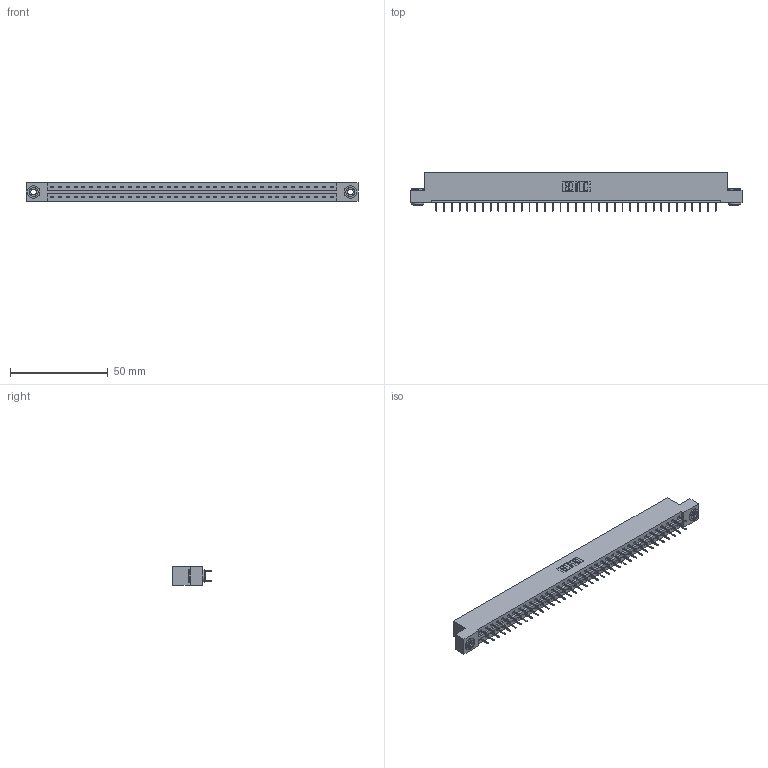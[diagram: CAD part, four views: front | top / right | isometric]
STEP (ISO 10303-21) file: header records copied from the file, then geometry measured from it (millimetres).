
FILE_DESCRIPTION (( 'STEP AP203' ), '1' );
FILE_NAME ('387-074-524-203.STEP', '2018-09-22T19:36:12', ( '' ), ( '' ), 'SwSTEP 2.0', 'SolidWorks 2016', '' );
FILE_SCHEMA (( 'CONFIG_CONTROL_DESIGN' ));
Length unit declared in the file: inch
Products named in the file (4): 337 Part_Flush Mounting Lugs - 0.156 Dia-TH; 345-292-001_345-293-124; 345-250-002_345-250-002-102; 387-074-524-203
Assembly tree (77 placements, depth 2):
  387-074-524-203
    337 Part_Flush Mounting Lugs - 0.156 Dia-TH
    345-292-001_345-293-124  x74
    345-250-002_345-250-002-102  x2
Bounding box: 169.62 x 19.69 x 9.4 mm (x, y, z)
Volume: 17716.9 mm3; surface area: 19858 mm2
Topology: 77 solids, 77 shells, 4444 faces, 12597 edges, 8098 vertices
Faces by surface type: plane 3336, cylinder 1100, cone 8
Entity records: 30058 total; most frequent: CARTESIAN_POINT 5041, ORIENTED_EDGE 4970, DIRECTION 4331, EDGE_CURVE 2485, VECTOR 2337, LINE 2337, VERTEX_POINT 1650, AXIS2_PLACEMENT_3D 997
